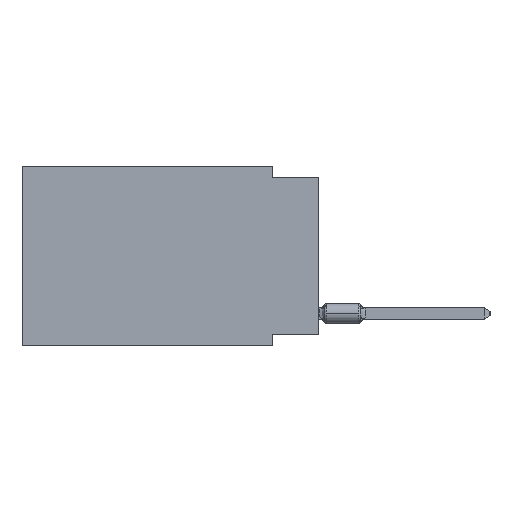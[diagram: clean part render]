
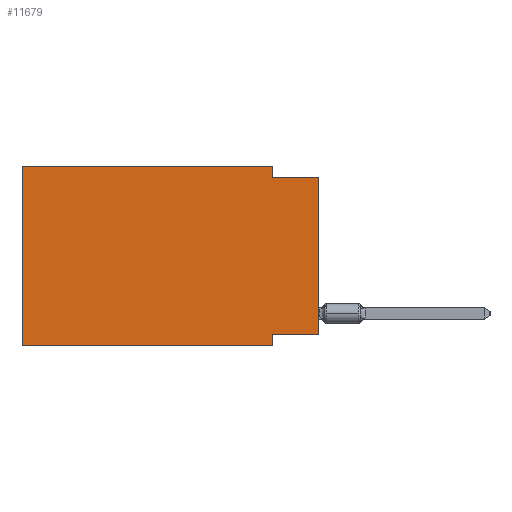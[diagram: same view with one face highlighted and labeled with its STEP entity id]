
A CAD part, left-side view. The second image highlights one B-rep face of the part: STEP entity #11679.
In plain terms, the highlighted planar face has unit normal (-1, 0, 0).
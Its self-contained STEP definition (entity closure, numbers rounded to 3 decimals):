
#1936 = EDGE_CURVE ( 'NONE', #19260, #37022, #15687, .T. ) ;
#2117 = LINE ( 'NONE', #8833, #21175 ) ;
#2912 = DIRECTION ( 'NONE',  ( 0., -1., 0. ) ) ;
#3073 = VECTOR ( 'NONE', #2912, 1000. ) ;
#4998 = CARTESIAN_POINT ( 'NONE',  ( 0., 2.54, -0.635 ) ) ;
#5229 = VERTEX_POINT ( 'NONE', #12611 ) ;
#5966 = LINE ( 'NONE', #30727, #3073 ) ;
#6436 = EDGE_CURVE ( 'NONE', #25938, #22444, #36866, .T. ) ;
#6989 = LINE ( 'NONE', #16352, #8829 ) ;
#8289 = ORIENTED_EDGE ( 'NONE', *, *, #9094, .F. ) ;
#8829 = VECTOR ( 'NONE', #12926, 1000. ) ;
#8833 = CARTESIAN_POINT ( 'NONE',  ( 0., 16.383, 0. ) ) ;
#8920 = VECTOR ( 'NONE', #21374, 1000. ) ;
#8957 = EDGE_CURVE ( 'NONE', #19260, #15203, #15945, .T. ) ;
#9094 = EDGE_CURVE ( 'NONE', #15203, #22444, #10844, .T. ) ;
#9688 = DIRECTION ( 'NONE',  ( 0., 0., -1. ) ) ;
#10165 = ORIENTED_EDGE ( 'NONE', *, *, #15822, .F. ) ;
#10666 = CARTESIAN_POINT ( 'NONE',  ( 0., 16.383, 0. ) ) ;
#10844 = LINE ( 'NONE', #16528, #16736 ) ;
#11679 = ADVANCED_FACE ( 'NONE', ( #31393 ), #18617, .F. ) ;
#11840 = CARTESIAN_POINT ( 'NONE',  ( 0., 0., 0. ) ) ;
#12611 = CARTESIAN_POINT ( 'NONE',  ( 0., 2.54, 0. ) ) ;
#12926 = DIRECTION ( 'NONE',  ( 0., -1., 0. ) ) ;
#15203 = VERTEX_POINT ( 'NONE', #39388 ) ;
#15687 = LINE ( 'NONE', #11840, #8920 ) ;
#15822 = EDGE_CURVE ( 'NONE', #5229, #21166, #29330, .T. ) ;
#15945 = LINE ( 'NONE', #16149, #33617 ) ;
#16149 = CARTESIAN_POINT ( 'NONE',  ( 0., 0., -9.271 ) ) ;
#16352 = CARTESIAN_POINT ( 'NONE',  ( 0., 0., -0.635 ) ) ;
#16528 = CARTESIAN_POINT ( 'NONE',  ( 0., 2.54, -9.906 ) ) ;
#16736 = VECTOR ( 'NONE', #28512, 1000. ) ;
#18184 = DIRECTION ( 'NONE',  ( 0., 0., 1. ) ) ;
#18271 = ORIENTED_EDGE ( 'NONE', *, *, #8957, .F. ) ;
#18582 = CARTESIAN_POINT ( 'NONE',  ( 0., 16.383, -9.906 ) ) ;
#18617 = PLANE ( 'NONE',  #27948 ) ;
#19260 = VERTEX_POINT ( 'NONE', #22333 ) ;
#19792 = CARTESIAN_POINT ( 'NONE',  ( 0., 2.54, 0. ) ) ;
#20200 = VERTEX_POINT ( 'NONE', #10666 ) ;
#21166 = VERTEX_POINT ( 'NONE', #4998 ) ;
#21175 = VECTOR ( 'NONE', #18184, 1000. ) ;
#21374 = DIRECTION ( 'NONE',  ( 0., 0., 1. ) ) ;
#22333 = CARTESIAN_POINT ( 'NONE',  ( 0., 0., -9.271 ) ) ;
#22444 = VERTEX_POINT ( 'NONE', #27088 ) ;
#22885 = ORIENTED_EDGE ( 'NONE', *, *, #34320, .F. ) ;
#24968 = CARTESIAN_POINT ( 'NONE',  ( 0., 0., -0.635 ) ) ;
#25092 = DIRECTION ( 'NONE',  ( 1., 0., 0. ) ) ;
#25938 = VERTEX_POINT ( 'NONE', #36167 ) ;
#26407 = ORIENTED_EDGE ( 'NONE', *, *, #27465, .F. ) ;
#26965 = VECTOR ( 'NONE', #33817, 1000. ) ;
#27072 = ORIENTED_EDGE ( 'NONE', *, *, #29526, .F. ) ;
#27088 = CARTESIAN_POINT ( 'NONE',  ( 0., 2.54, -9.906 ) ) ;
#27465 = EDGE_CURVE ( 'NONE', #21166, #37022, #6989, .T. ) ;
#27948 = AXIS2_PLACEMENT_3D ( 'NONE', #28143, #25092, #9688 ) ;
#28143 = CARTESIAN_POINT ( 'NONE',  ( 0., 16.383, 0. ) ) ;
#28512 = DIRECTION ( 'NONE',  ( 0., 0., -1. ) ) ;
#28724 = DIRECTION ( 'NONE',  ( 0., 0., -1. ) ) ;
#29330 = LINE ( 'NONE', #19792, #33666 ) ;
#29526 = EDGE_CURVE ( 'NONE', #20200, #5229, #5966, .T. ) ;
#29617 = ORIENTED_EDGE ( 'NONE', *, *, #6436, .T. ) ;
#29901 = EDGE_LOOP ( 'NONE', ( #38597, #26407, #10165, #27072, #22885, #29617, #8289, #18271 ) ) ;
#30727 = CARTESIAN_POINT ( 'NONE',  ( 0., 16.383, 0. ) ) ;
#31393 = FACE_OUTER_BOUND ( 'NONE', #29901, .T. ) ;
#33617 = VECTOR ( 'NONE', #39917, 1000. ) ;
#33666 = VECTOR ( 'NONE', #28724, 1000. ) ;
#33817 = DIRECTION ( 'NONE',  ( 0., -1., 0. ) ) ;
#34320 = EDGE_CURVE ( 'NONE', #25938, #20200, #2117, .T. ) ;
#36167 = CARTESIAN_POINT ( 'NONE',  ( 0., 16.383, -9.906 ) ) ;
#36866 = LINE ( 'NONE', #18582, #26965 ) ;
#37022 = VERTEX_POINT ( 'NONE', #24968 ) ;
#38597 = ORIENTED_EDGE ( 'NONE', *, *, #1936, .T. ) ;
#39388 = CARTESIAN_POINT ( 'NONE',  ( 0., 2.54, -9.271 ) ) ;
#39917 = DIRECTION ( 'NONE',  ( 0., 1., 0. ) ) ;
